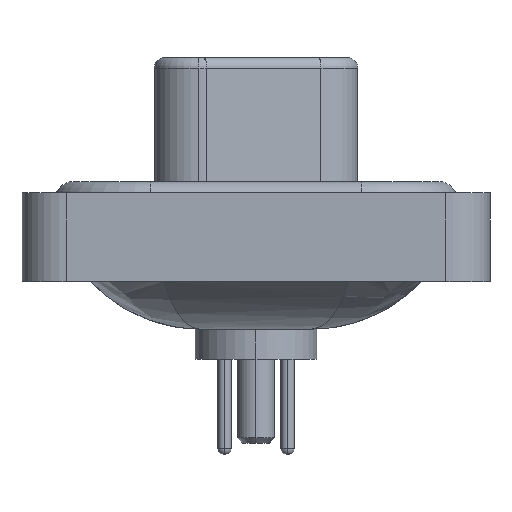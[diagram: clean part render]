
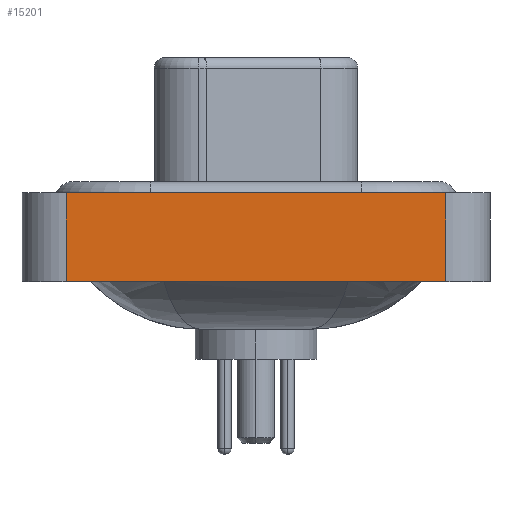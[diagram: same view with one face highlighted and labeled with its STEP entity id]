
A CAD part, left-side view. The second image highlights one B-rep face of the part: STEP entity #15201.
In plain terms, the highlighted planar face has unit normal (-1, 0, 0).
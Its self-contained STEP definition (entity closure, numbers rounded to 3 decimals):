
#40 = EDGE_CURVE ( 'NONE', #17723, #12571, #5028, .T. ) ;
#364 = DIRECTION ( 'NONE',  ( -1., 0., 0. ) ) ;
#1147 = DIRECTION ( 'NONE',  ( 0., -1., 0. ) ) ;
#1974 = EDGE_CURVE ( 'NONE', #12680, #17723, #5551, .T. ) ;
#2102 = DIRECTION ( 'NONE',  ( 0., 0., 1. ) ) ;
#2145 = CARTESIAN_POINT ( 'NONE',  ( -7.35, 8.55, -3.6 ) ) ;
#2481 = ORIENTED_EDGE ( 'NONE', *, *, #1974, .T. ) ;
#2793 = VERTEX_POINT ( 'NONE', #16263 ) ;
#3011 = CARTESIAN_POINT ( 'NONE',  ( -7.35, -8.55, 0.4 ) ) ;
#3221 = CARTESIAN_POINT ( 'NONE',  ( -7.35, -8.55, -3.6 ) ) ;
#4680 = DIRECTION ( 'NONE',  ( 0., 0., 1. ) ) ;
#4816 = LINE ( 'NONE', #17675, #17492 ) ;
#5028 = LINE ( 'NONE', #17902, #9702 ) ;
#5551 = LINE ( 'NONE', #16947, #16468 ) ;
#5949 = LINE ( 'NONE', #3011, #15461 ) ;
#6018 = CARTESIAN_POINT ( 'NONE',  ( -7.35, -8.55, 0.4 ) ) ;
#7855 = ORIENTED_EDGE ( 'NONE', *, *, #16362, .F. ) ;
#8663 = DIRECTION ( 'NONE',  ( 0., -1., 0. ) ) ;
#9702 = VECTOR ( 'NONE', #2102, 1000. ) ;
#9896 = FACE_OUTER_BOUND ( 'NONE', #14886, .T. ) ;
#10191 = EDGE_CURVE ( 'NONE', #12680, #2793, #4816, .T. ) ;
#11100 = CARTESIAN_POINT ( 'NONE',  ( -7.35, -8.55, -3.6 ) ) ;
#12571 = VERTEX_POINT ( 'NONE', #6018 ) ;
#12680 = VERTEX_POINT ( 'NONE', #2145 ) ;
#13787 = AXIS2_PLACEMENT_3D ( 'NONE', #3221, #364, #4680 ) ;
#13957 = ORIENTED_EDGE ( 'NONE', *, *, #40, .T. ) ;
#14732 = PLANE ( 'NONE',  #13787 ) ;
#14886 = EDGE_LOOP ( 'NONE', ( #13957, #7855, #19654, #2481 ) ) ;
#15201 = ADVANCED_FACE ( 'NONE', ( #9896 ), #14732, .T. ) ;
#15461 = VECTOR ( 'NONE', #1147, 1000. ) ;
#15720 = DIRECTION ( 'NONE',  ( 0., 0., 1. ) ) ;
#16263 = CARTESIAN_POINT ( 'NONE',  ( -7.35, 8.55, 0.4 ) ) ;
#16362 = EDGE_CURVE ( 'NONE', #2793, #12571, #5949, .T. ) ;
#16468 = VECTOR ( 'NONE', #8663, 1000. ) ;
#16947 = CARTESIAN_POINT ( 'NONE',  ( -7.35, -8.55, -3.6 ) ) ;
#17492 = VECTOR ( 'NONE', #15720, 1000. ) ;
#17675 = CARTESIAN_POINT ( 'NONE',  ( -7.35, 8.55, -3.6 ) ) ;
#17723 = VERTEX_POINT ( 'NONE', #11100 ) ;
#17902 = CARTESIAN_POINT ( 'NONE',  ( -7.35, -8.55, -3.6 ) ) ;
#19654 = ORIENTED_EDGE ( 'NONE', *, *, #10191, .F. ) ;
